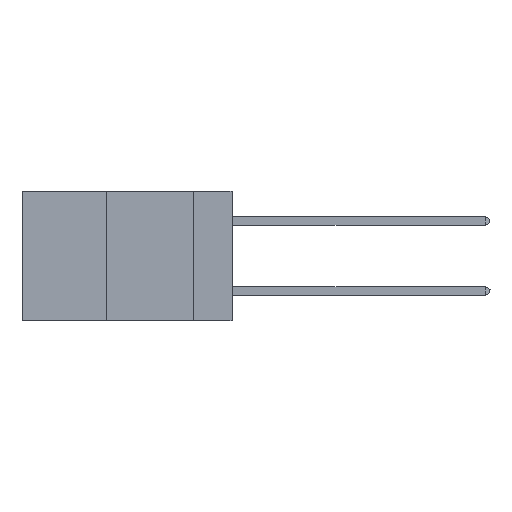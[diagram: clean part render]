
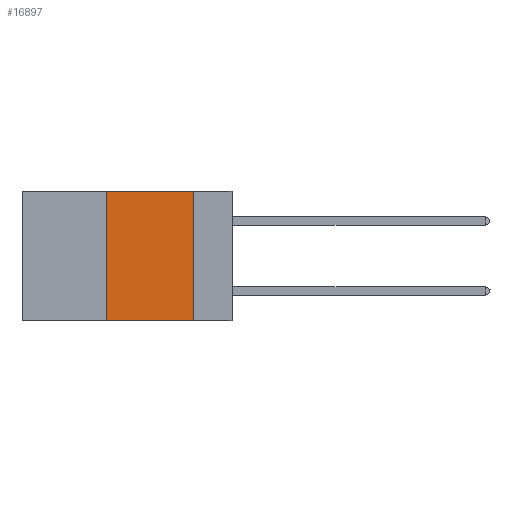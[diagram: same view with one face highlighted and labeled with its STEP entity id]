
A CAD part, left-side view. The second image highlights one B-rep face of the part: STEP entity #16897.
In plain terms, the highlighted planar face has unit normal (-1, 0, 0).
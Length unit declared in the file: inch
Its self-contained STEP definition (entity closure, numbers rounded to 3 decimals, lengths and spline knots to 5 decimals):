
#1486 = CARTESIAN_POINT ( 'NONE',  ( 0., 0.6, 0. ) ) ;
#1637 = DIRECTION ( 'NONE',  ( 1., 0., 0. ) ) ;
#1730 = VERTEX_POINT ( 'NONE', #8353 ) ;
#2143 = CARTESIAN_POINT ( 'NONE',  ( 0., 0.36, -0.37 ) ) ;
#5031 = CARTESIAN_POINT ( 'NONE',  ( 0., 0.36, 0. ) ) ;
#5547 = ORIENTED_EDGE ( 'NONE', *, *, #7126, .F. ) ;
#6205 = LINE ( 'NONE', #30860, #10994 ) ;
#7126 = EDGE_CURVE ( 'NONE', #10394, #23981, #6205, .T. ) ;
#8256 = VECTOR ( 'NONE', #20986, 39.37008 ) ;
#8290 = VECTOR ( 'NONE', #9555, 39.37008 ) ;
#8353 = CARTESIAN_POINT ( 'NONE',  ( 0., 0.11, -0.37 ) ) ;
#8366 = AXIS2_PLACEMENT_3D ( 'NONE', #1486, #1637, #21778 ) ;
#9086 = DIRECTION ( 'NONE',  ( 0., -1., 0. ) ) ;
#9555 = DIRECTION ( 'NONE',  ( 0., -1., 0. ) ) ;
#9639 = EDGE_CURVE ( 'NONE', #19991, #10394, #29041, .T. ) ;
#10394 = VERTEX_POINT ( 'NONE', #26061 ) ;
#10994 = VECTOR ( 'NONE', #9086, 39.37008 ) ;
#11003 = EDGE_LOOP ( 'NONE', ( #17871, #5547, #14593, #23905 ) ) ;
#11032 = CARTESIAN_POINT ( 'NONE',  ( 0., 0.11, 0. ) ) ;
#13683 = LINE ( 'NONE', #17979, #8256 ) ;
#14464 = FACE_OUTER_BOUND ( 'NONE', #11003, .T. ) ;
#14593 = ORIENTED_EDGE ( 'NONE', *, *, #9639, .F. ) ;
#15504 = EDGE_CURVE ( 'NONE', #19991, #1730, #28462, .T. ) ;
#16079 = PLANE ( 'NONE',  #8366 ) ;
#16897 = ADVANCED_FACE ( 'NONE', ( #14464 ), #16079, .F. ) ;
#17871 = ORIENTED_EDGE ( 'NONE', *, *, #24383, .F. ) ;
#17979 = CARTESIAN_POINT ( 'NONE',  ( 0., 0.11, 0. ) ) ;
#19991 = VERTEX_POINT ( 'NONE', #2143 ) ;
#20986 = DIRECTION ( 'NONE',  ( 0., 0., -1. ) ) ;
#21560 = VECTOR ( 'NONE', #24419, 39.37008 ) ;
#21778 = DIRECTION ( 'NONE',  ( 0., 0., -1. ) ) ;
#23905 = ORIENTED_EDGE ( 'NONE', *, *, #15504, .T. ) ;
#23981 = VERTEX_POINT ( 'NONE', #11032 ) ;
#24383 = EDGE_CURVE ( 'NONE', #23981, #1730, #13683, .T. ) ;
#24419 = DIRECTION ( 'NONE',  ( 0., 0., 1. ) ) ;
#26061 = CARTESIAN_POINT ( 'NONE',  ( 0., 0.36, 0. ) ) ;
#28462 = LINE ( 'NONE', #31326, #8290 ) ;
#29041 = LINE ( 'NONE', #5031, #21560 ) ;
#30860 = CARTESIAN_POINT ( 'NONE',  ( 0., 0.6, 0. ) ) ;
#31326 = CARTESIAN_POINT ( 'NONE',  ( 0., 0.6, -0.37 ) ) ;
